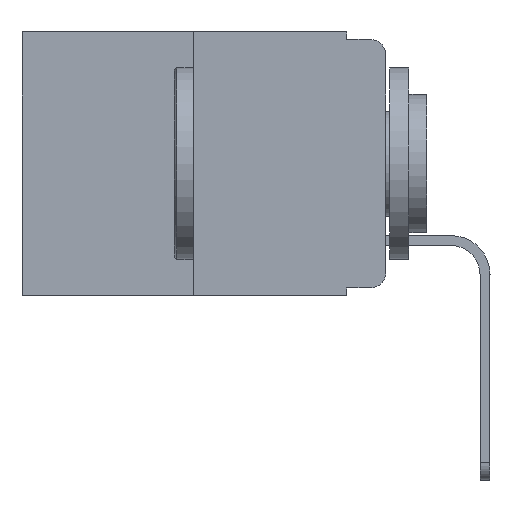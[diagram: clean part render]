
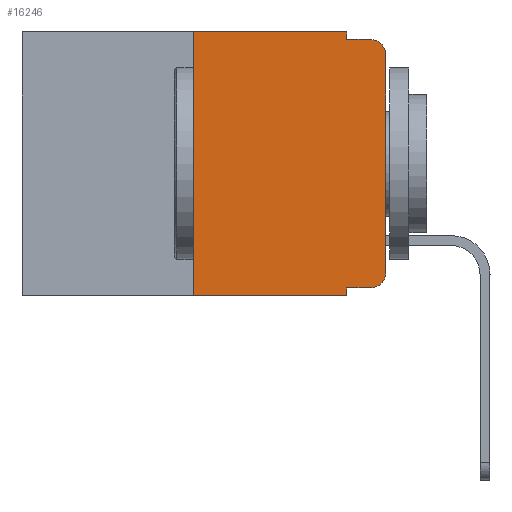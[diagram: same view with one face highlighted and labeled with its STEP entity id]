
A CAD part, left-side view. The second image highlights one B-rep face of the part: STEP entity #16246.
In plain terms, the highlighted planar face has unit normal (-1, 0, 0).
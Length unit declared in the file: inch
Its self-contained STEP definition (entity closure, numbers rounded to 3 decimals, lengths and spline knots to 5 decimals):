
#164 = ORIENTED_EDGE ( 'NONE', *, *, #16788, .T. ) ;
#211 = CARTESIAN_POINT ( 'NONE',  ( 0., 0.02, -0.313 ) ) ;
#262 = ORIENTED_EDGE ( 'NONE', *, *, #12639, .F. ) ;
#610 = EDGE_CURVE ( 'NONE', #6276, #8563, #23240, .T. ) ;
#835 = EDGE_LOOP ( 'NONE', ( #23334, #18271, #262, #2453, #4418, #10681, #3629, #3614, #164, #21155 ) ) ;
#1376 = EDGE_CURVE ( 'NONE', #8563, #7350, #12734, .T. ) ;
#1436 = LINE ( 'NONE', #3594, #7115 ) ;
#1795 = DIRECTION ( 'NONE',  ( -1., 0., 0. ) ) ;
#1810 = EDGE_CURVE ( 'NONE', #23299, #17759, #21629, .T. ) ;
#1812 = LINE ( 'NONE', #8763, #4800 ) ;
#1975 = VECTOR ( 'NONE', #16390, 39.37008 ) ;
#2048 = VERTEX_POINT ( 'NONE', #20461 ) ;
#2453 = ORIENTED_EDGE ( 'NONE', *, *, #10283, .F. ) ;
#3318 = LINE ( 'NONE', #8753, #6898 ) ;
#3351 = CARTESIAN_POINT ( 'NONE',  ( 0., 0.051, -0.01 ) ) ;
#3594 = CARTESIAN_POINT ( 'NONE',  ( 0., 0.051, 0. ) ) ;
#3614 = ORIENTED_EDGE ( 'NONE', *, *, #11783, .F. ) ;
#3629 = ORIENTED_EDGE ( 'NONE', *, *, #14163, .T. ) ;
#4149 = AXIS2_PLACEMENT_3D ( 'NONE', #211, #17408, #23619 ) ;
#4174 = VERTEX_POINT ( 'NONE', #20205 ) ;
#4321 = DIRECTION ( 'NONE',  ( 0., 0., -1. ) ) ;
#4418 = ORIENTED_EDGE ( 'NONE', *, *, #8175, .F. ) ;
#4800 = VECTOR ( 'NONE', #10698, 39.37008 ) ;
#5002 = FACE_OUTER_BOUND ( 'NONE', #835, .T. ) ;
#5295 = CARTESIAN_POINT ( 'NONE',  ( 0., 0.473, 0. ) ) ;
#5682 = DIRECTION ( 'NONE',  ( 0., 0., -1. ) ) ;
#5772 = CARTESIAN_POINT ( 'NONE',  ( 0., 0.25, -0.343 ) ) ;
#6276 = VERTEX_POINT ( 'NONE', #15050 ) ;
#6792 = CARTESIAN_POINT ( 'NONE',  ( 0., 0., 0. ) ) ;
#6894 = VERTEX_POINT ( 'NONE', #3351 ) ;
#6898 = VECTOR ( 'NONE', #24198, 39.37008 ) ;
#6922 = DIRECTION ( 'NONE',  ( 1., 0., 0. ) ) ;
#7115 = VECTOR ( 'NONE', #5682, 39.37008 ) ;
#7225 = LINE ( 'NONE', #12614, #9621 ) ;
#7350 = VERTEX_POINT ( 'NONE', #17681 ) ;
#7905 = CARTESIAN_POINT ( 'NONE',  ( 0., 0.051, 0. ) ) ;
#8175 = EDGE_CURVE ( 'NONE', #17759, #23841, #3318, .T. ) ;
#8563 = VERTEX_POINT ( 'NONE', #20866 ) ;
#8673 = DIRECTION ( 'NONE',  ( 0., 0., 1. ) ) ;
#8753 = CARTESIAN_POINT ( 'NONE',  ( 0., 0.473, 0. ) ) ;
#8763 = CARTESIAN_POINT ( 'NONE',  ( 0., 0.473, -0.343 ) ) ;
#9422 = LINE ( 'NONE', #7905, #23433 ) ;
#9621 = VECTOR ( 'NONE', #20284, 39.37008 ) ;
#10283 = EDGE_CURVE ( 'NONE', #23841, #6894, #1436, .T. ) ;
#10325 = VECTOR ( 'NONE', #14419, 39.37008 ) ;
#10681 = ORIENTED_EDGE ( 'NONE', *, *, #1810, .F. ) ;
#10698 = DIRECTION ( 'NONE',  ( 0., -1., 0. ) ) ;
#10819 = CARTESIAN_POINT ( 'NONE',  ( 0., 0.051, 0. ) ) ;
#10866 = PLANE ( 'NONE',  #17979 ) ;
#11019 = AXIS2_PLACEMENT_3D ( 'NONE', #11302, #1795, #13036 ) ;
#11302 = CARTESIAN_POINT ( 'NONE',  ( 0., 0.02, -0.03 ) ) ;
#11499 = CARTESIAN_POINT ( 'NONE',  ( 0., 0.25, 0. ) ) ;
#11783 = EDGE_CURVE ( 'NONE', #2048, #24166, #9422, .T. ) ;
#11973 = DIRECTION ( 'NONE',  ( 0., 0., -1. ) ) ;
#12574 = CARTESIAN_POINT ( 'NONE',  ( 0., 0.25, 0. ) ) ;
#12614 = CARTESIAN_POINT ( 'NONE',  ( 0., 0.051, -0.01 ) ) ;
#12639 = EDGE_CURVE ( 'NONE', #6894, #4174, #7225, .T. ) ;
#12734 = LINE ( 'NONE', #6792, #13937 ) ;
#13036 = DIRECTION ( 'NONE',  ( 0., 0., -1. ) ) ;
#13937 = VECTOR ( 'NONE', #8673, 39.37008 ) ;
#14163 = EDGE_CURVE ( 'NONE', #23299, #24166, #1812, .T. ) ;
#14419 = DIRECTION ( 'NONE',  ( 0., -1., 0. ) ) ;
#15050 = CARTESIAN_POINT ( 'NONE',  ( 0., 0.02, -0.333 ) ) ;
#15364 = LINE ( 'NONE', #18072, #10325 ) ;
#16246 = ADVANCED_FACE ( 'NONE', ( #5002 ), #10866, .F. ) ;
#16390 = DIRECTION ( 'NONE',  ( 0., 0., 1. ) ) ;
#16788 = EDGE_CURVE ( 'NONE', #2048, #6276, #15364, .T. ) ;
#17267 = CARTESIAN_POINT ( 'NONE',  ( 0., 0.051, -0.343 ) ) ;
#17408 = DIRECTION ( 'NONE',  ( -1., 0., 0. ) ) ;
#17681 = CARTESIAN_POINT ( 'NONE',  ( 0., 0., -0.03 ) ) ;
#17759 = VERTEX_POINT ( 'NONE', #11499 ) ;
#17979 = AXIS2_PLACEMENT_3D ( 'NONE', #5295, #6922, #4321 ) ;
#18072 = CARTESIAN_POINT ( 'NONE',  ( 0., 0.051, -0.333 ) ) ;
#18265 = EDGE_CURVE ( 'NONE', #7350, #4174, #21276, .T. ) ;
#18271 = ORIENTED_EDGE ( 'NONE', *, *, #18265, .T. ) ;
#20205 = CARTESIAN_POINT ( 'NONE',  ( 0., 0.02, -0.01 ) ) ;
#20284 = DIRECTION ( 'NONE',  ( 0., -1., 0. ) ) ;
#20461 = CARTESIAN_POINT ( 'NONE',  ( 0., 0.051, -0.333 ) ) ;
#20866 = CARTESIAN_POINT ( 'NONE',  ( 0., 0., -0.313 ) ) ;
#21155 = ORIENTED_EDGE ( 'NONE', *, *, #610, .T. ) ;
#21276 = CIRCLE ( 'NONE', #11019, 0.02 ) ;
#21629 = LINE ( 'NONE', #12574, #1975 ) ;
#23240 = CIRCLE ( 'NONE', #4149, 0.02 ) ;
#23299 = VERTEX_POINT ( 'NONE', #5772 ) ;
#23334 = ORIENTED_EDGE ( 'NONE', *, *, #1376, .T. ) ;
#23433 = VECTOR ( 'NONE', #11973, 39.37008 ) ;
#23619 = DIRECTION ( 'NONE',  ( 0., 0., -1. ) ) ;
#23841 = VERTEX_POINT ( 'NONE', #10819 ) ;
#24166 = VERTEX_POINT ( 'NONE', #17267 ) ;
#24198 = DIRECTION ( 'NONE',  ( 0., -1., 0. ) ) ;
